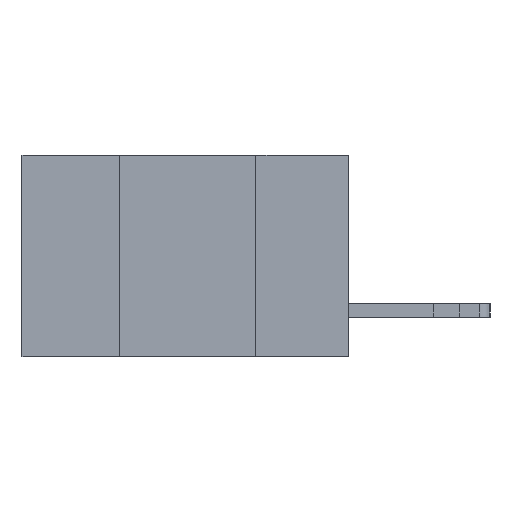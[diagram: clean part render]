
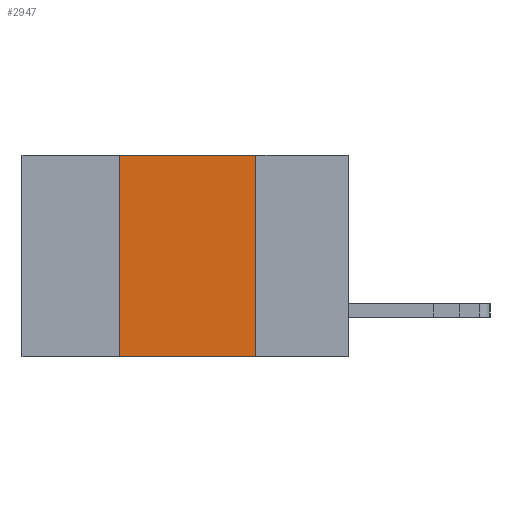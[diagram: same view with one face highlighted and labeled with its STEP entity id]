
A CAD part, left-side view. The second image highlights one B-rep face of the part: STEP entity #2947.
In plain terms, the highlighted planar face has unit normal (-1, 0, 0).
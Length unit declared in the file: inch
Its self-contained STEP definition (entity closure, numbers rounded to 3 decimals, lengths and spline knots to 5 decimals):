
#432 = DIRECTION ( 'NONE',  ( 0., -1., 0. ) ) ;
#1222 = VERTEX_POINT ( 'NONE', #9683 ) ;
#1763 = EDGE_LOOP ( 'NONE', ( #7804, #12910, #12535, #11596 ) ) ;
#1867 = VECTOR ( 'NONE', #18417, 39.37008 ) ;
#1869 = DIRECTION ( 'NONE',  ( 0., 0., -1. ) ) ;
#1969 = DIRECTION ( 'NONE',  ( 1., 0., 0. ) ) ;
#2269 = VERTEX_POINT ( 'NONE', #18231 ) ;
#2619 = VERTEX_POINT ( 'NONE', #11895 ) ;
#2947 = ADVANCED_FACE ( 'NONE', ( #16553 ), #3247, .F. ) ;
#3247 = PLANE ( 'NONE',  #15538 ) ;
#3410 = CARTESIAN_POINT ( 'NONE',  ( 0., 0.6, 0. ) ) ;
#3931 = CARTESIAN_POINT ( 'NONE',  ( 0., 0.42, 0. ) ) ;
#4528 = VECTOR ( 'NONE', #432, 39.37008 ) ;
#4558 = CARTESIAN_POINT ( 'NONE',  ( 0., 0.17, -0.37 ) ) ;
#5025 = VECTOR ( 'NONE', #14692, 39.37008 ) ;
#5441 = CARTESIAN_POINT ( 'NONE',  ( 0., 0.6, -0.37 ) ) ;
#6184 = LINE ( 'NONE', #16874, #1867 ) ;
#7804 = ORIENTED_EDGE ( 'NONE', *, *, #14436, .F. ) ;
#9199 = LINE ( 'NONE', #9979, #4528 ) ;
#9683 = CARTESIAN_POINT ( 'NONE',  ( 0., 0.42, -0.37 ) ) ;
#9979 = CARTESIAN_POINT ( 'NONE',  ( 0., 0.6, 0. ) ) ;
#10722 = LINE ( 'NONE', #3931, #19335 ) ;
#11596 = ORIENTED_EDGE ( 'NONE', *, *, #17542, .T. ) ;
#11895 = CARTESIAN_POINT ( 'NONE',  ( 0., 0.42, 0. ) ) ;
#12018 = EDGE_CURVE ( 'NONE', #2619, #2269, #9199, .T. ) ;
#12535 = ORIENTED_EDGE ( 'NONE', *, *, #16488, .F. ) ;
#12910 = ORIENTED_EDGE ( 'NONE', *, *, #12018, .F. ) ;
#13266 = DIRECTION ( 'NONE',  ( 0., 0., 1. ) ) ;
#13286 = LINE ( 'NONE', #5441, #5025 ) ;
#14436 = EDGE_CURVE ( 'NONE', #2269, #18150, #6184, .T. ) ;
#14692 = DIRECTION ( 'NONE',  ( 0., -1., 0. ) ) ;
#15538 = AXIS2_PLACEMENT_3D ( 'NONE', #3410, #1969, #1869 ) ;
#16488 = EDGE_CURVE ( 'NONE', #1222, #2619, #10722, .T. ) ;
#16553 = FACE_OUTER_BOUND ( 'NONE', #1763, .T. ) ;
#16874 = CARTESIAN_POINT ( 'NONE',  ( 0., 0.17, 0. ) ) ;
#17542 = EDGE_CURVE ( 'NONE', #1222, #18150, #13286, .T. ) ;
#18150 = VERTEX_POINT ( 'NONE', #4558 ) ;
#18231 = CARTESIAN_POINT ( 'NONE',  ( 0., 0.17, 0. ) ) ;
#18417 = DIRECTION ( 'NONE',  ( 0., 0., -1. ) ) ;
#19335 = VECTOR ( 'NONE', #13266, 39.37008 ) ;
